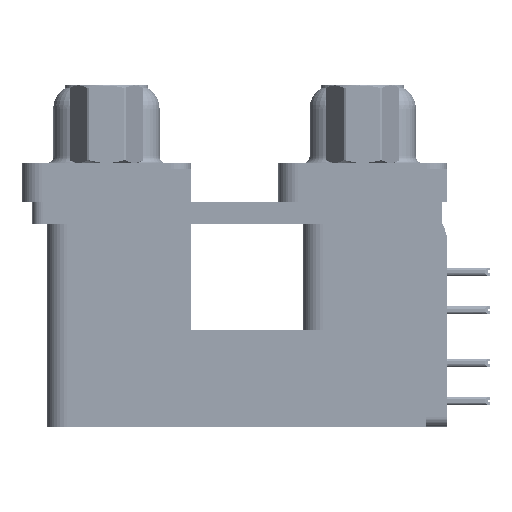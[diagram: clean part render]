
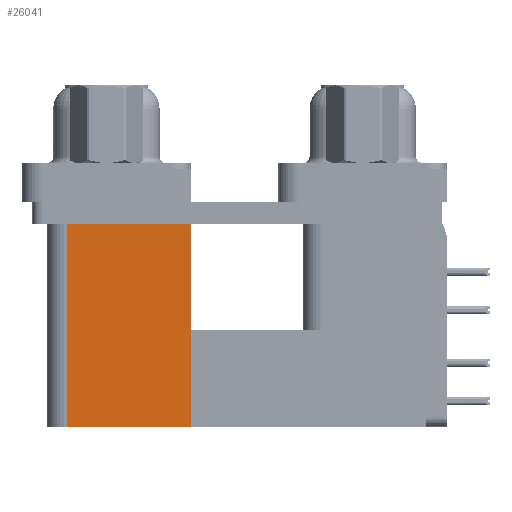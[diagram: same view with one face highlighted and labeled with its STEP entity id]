
A CAD part, left-side view. The second image highlights one B-rep face of the part: STEP entity #26041.
In plain terms, the highlighted planar face has unit normal (-1, 0, 0).
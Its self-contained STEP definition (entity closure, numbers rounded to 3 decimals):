
#1640 = PLANE ( 'NONE',  #20252 ) ;
#2190 = DIRECTION ( 'NONE',  ( 0., 0., -1. ) ) ;
#2232 = DIRECTION ( 'NONE',  ( 0., 0., 1. ) ) ;
#5356 = LINE ( 'NONE', #39227, #16321 ) ;
#6476 = EDGE_LOOP ( 'NONE', ( #40947, #22461, #7731, #18995 ) ) ;
#7156 = EDGE_CURVE ( 'NONE', #32007, #13868, #5356, .T. ) ;
#7731 = ORIENTED_EDGE ( 'NONE', *, *, #7156, .F. ) ;
#10518 = DIRECTION ( 'NONE',  ( 0., 1., 0. ) ) ;
#11182 = LINE ( 'NONE', #44251, #25527 ) ;
#13868 = VERTEX_POINT ( 'NONE', #37094 ) ;
#15828 = CARTESIAN_POINT ( 'NONE',  ( 3.765, 12.775, -19.2 ) ) ;
#16321 = VECTOR ( 'NONE', #10518, 1000. ) ;
#18995 = ORIENTED_EDGE ( 'NONE', *, *, #32401, .T. ) ;
#20166 = VERTEX_POINT ( 'NONE', #47565 ) ;
#20252 = AXIS2_PLACEMENT_3D ( 'NONE', #47491, #30930, #2190 ) ;
#22311 = VECTOR ( 'NONE', #49481, 1000. ) ;
#22461 = ORIENTED_EDGE ( 'NONE', *, *, #48242, .F. ) ;
#24174 = DIRECTION ( 'NONE',  ( 0., 1., 0. ) ) ;
#25527 = VECTOR ( 'NONE', #24174, 1000. ) ;
#26041 = ADVANCED_FACE ( 'NONE', ( #51282 ), #1640, .F. ) ;
#27734 = CARTESIAN_POINT ( 'NONE',  ( 3.765, 12.775, -2.5 ) ) ;
#30930 = DIRECTION ( 'NONE',  ( 1., 0., 0. ) ) ;
#30972 = CARTESIAN_POINT ( 'NONE',  ( 3.765, 12.775, -19.2 ) ) ;
#32007 = VERTEX_POINT ( 'NONE', #15828 ) ;
#32401 = EDGE_CURVE ( 'NONE', #32007, #33021, #35018, .T. ) ;
#33021 = VERTEX_POINT ( 'NONE', #27734 ) ;
#33186 = CARTESIAN_POINT ( 'NONE',  ( 3.765, 21.975, -19.2 ) ) ;
#35018 = LINE ( 'NONE', #30972, #51032 ) ;
#37094 = CARTESIAN_POINT ( 'NONE',  ( 3.765, 21.975, -19.2 ) ) ;
#39227 = CARTESIAN_POINT ( 'NONE',  ( 3.765, 12.775, -19.2 ) ) ;
#40947 = ORIENTED_EDGE ( 'NONE', *, *, #52858, .T. ) ;
#44251 = CARTESIAN_POINT ( 'NONE',  ( 3.765, 12.775, -2.5 ) ) ;
#45962 = LINE ( 'NONE', #33186, #22311 ) ;
#47491 = CARTESIAN_POINT ( 'NONE',  ( 3.765, 12.775, -19.2 ) ) ;
#47565 = CARTESIAN_POINT ( 'NONE',  ( 3.765, 21.975, -2.5 ) ) ;
#48242 = EDGE_CURVE ( 'NONE', #13868, #20166, #45962, .T. ) ;
#49481 = DIRECTION ( 'NONE',  ( 0., 0., 1. ) ) ;
#51032 = VECTOR ( 'NONE', #2232, 1000. ) ;
#51282 = FACE_OUTER_BOUND ( 'NONE', #6476, .T. ) ;
#52858 = EDGE_CURVE ( 'NONE', #33021, #20166, #11182, .T. ) ;
